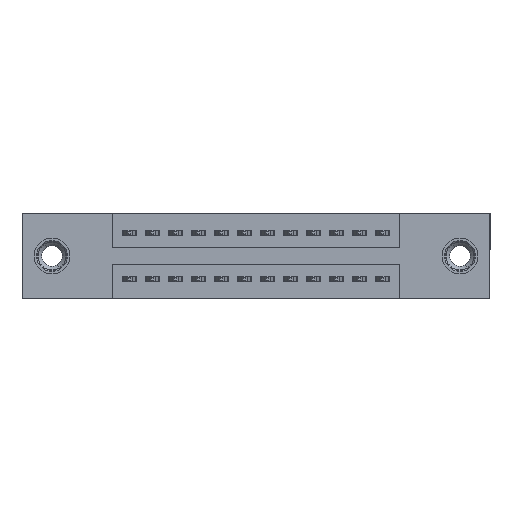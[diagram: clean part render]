
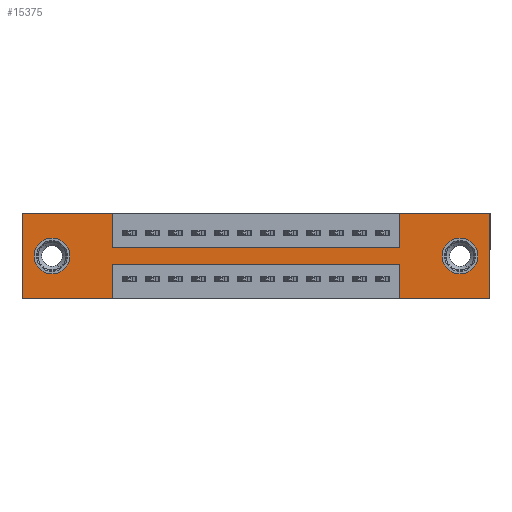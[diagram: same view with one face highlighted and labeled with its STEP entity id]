
A CAD part, front view. The second image highlights one B-rep face of the part: STEP entity #15375.
In plain terms, the highlighted planar face has unit normal (0, -1, 0).
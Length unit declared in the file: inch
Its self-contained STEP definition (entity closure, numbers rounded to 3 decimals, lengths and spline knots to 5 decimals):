
#65 = DIRECTION ( 'NONE',  ( -1., 0., 0. ) ) ;
#118 = ORIENTED_EDGE ( 'NONE', *, *, #15024, .F. ) ;
#172 = AXIS2_PLACEMENT_3D ( 'NONE', #2912, #1698, #9025 ) ;
#315 = VECTOR ( 'NONE', #1634, 39.37008 ) ;
#339 = VERTEX_POINT ( 'NONE', #6235 ) ;
#439 = ORIENTED_EDGE ( 'NONE', *, *, #13453, .T. ) ;
#585 = EDGE_CURVE ( 'NONE', #5337, #15615, #1363, .T. ) ;
#677 = DIRECTION ( 'NONE',  ( 0., 1., 0. ) ) ;
#715 = DIRECTION ( 'NONE',  ( 0., -1., 0. ) ) ;
#903 = VERTEX_POINT ( 'NONE', #2803 ) ;
#1064 = VERTEX_POINT ( 'NONE', #2848 ) ;
#1244 = ORIENTED_EDGE ( 'NONE', *, *, #11249, .F. ) ;
#1256 = LINE ( 'NONE', #8473, #9997 ) ;
#1363 = CIRCLE ( 'NONE', #172, 0.078 ) ;
#1538 = VECTOR ( 'NONE', #12690, 39.37008 ) ;
#1634 = DIRECTION ( 'NONE',  ( -1., 0., 0. ) ) ;
#1678 = CARTESIAN_POINT ( 'NONE',  ( 0.13, 0., -0.185 ) ) ;
#1698 = DIRECTION ( 'NONE',  ( 0., 1., 0. ) ) ;
#1923 = DIRECTION ( 'NONE',  ( 0., 0., -1. ) ) ;
#1973 = EDGE_CURVE ( 'NONE', #9704, #10598, #13847, .T. ) ;
#2004 = VERTEX_POINT ( 'NONE', #6261 ) ;
#2023 = ORIENTED_EDGE ( 'NONE', *, *, #9895, .F. ) ;
#2038 = LINE ( 'NONE', #3874, #14776 ) ;
#2069 = CARTESIAN_POINT ( 'NONE',  ( 0.3925, 0., 0. ) ) ;
#2102 = VECTOR ( 'NONE', #7076, 39.37008 ) ;
#2186 = EDGE_LOOP ( 'NONE', ( #14781, #3223 ) ) ;
#2247 = VECTOR ( 'NONE', #9769, 39.37008 ) ;
#2289 = DIRECTION ( 'NONE',  ( 0., 0., -1. ) ) ;
#2342 = CARTESIAN_POINT ( 'NONE',  ( 0., 0., 0. ) ) ;
#2355 = VERTEX_POINT ( 'NONE', #6116 ) ;
#2509 = VERTEX_POINT ( 'NONE', #3769 ) ;
#2595 = DIRECTION ( 'NONE',  ( 0., 0., 1. ) ) ;
#2657 = FACE_BOUND ( 'NONE', #2186, .T. ) ;
#2741 = CARTESIAN_POINT ( 'NONE',  ( 0.3925, 0., -0.22 ) ) ;
#2803 = CARTESIAN_POINT ( 'NONE',  ( 2.035, 0., 0. ) ) ;
#2838 = ORIENTED_EDGE ( 'NONE', *, *, #7203, .F. ) ;
#2848 = CARTESIAN_POINT ( 'NONE',  ( 1.6425, 0., -0.37 ) ) ;
#2882 = DIRECTION ( 'NONE',  ( 0., 0., 1. ) ) ;
#2912 = CARTESIAN_POINT ( 'NONE',  ( 1.905, 0., -0.185 ) ) ;
#3102 = DIRECTION ( 'NONE',  ( 0., 0., -1. ) ) ;
#3210 = CARTESIAN_POINT ( 'NONE',  ( 1.905, 0., -0.107 ) ) ;
#3223 = ORIENTED_EDGE ( 'NONE', *, *, #9840, .T. ) ;
#3570 = CARTESIAN_POINT ( 'NONE',  ( 0.3925, 0., -0.15 ) ) ;
#3715 = VERTEX_POINT ( 'NONE', #8625 ) ;
#3760 = LINE ( 'NONE', #9554, #12488 ) ;
#3769 = CARTESIAN_POINT ( 'NONE',  ( 0., 0., -0.37 ) ) ;
#3874 = CARTESIAN_POINT ( 'NONE',  ( 0.3925, 0., 0. ) ) ;
#4836 = CARTESIAN_POINT ( 'NONE',  ( 0.13, 0., -0.185 ) ) ;
#4933 = ORIENTED_EDGE ( 'NONE', *, *, #10602, .F. ) ;
#5054 = LINE ( 'NONE', #15081, #10585 ) ;
#5174 = CARTESIAN_POINT ( 'NONE',  ( 1.6425, 0., 0. ) ) ;
#5337 = VERTEX_POINT ( 'NONE', #3210 ) ;
#5484 = VECTOR ( 'NONE', #6401, 39.37008 ) ;
#5520 = VERTEX_POINT ( 'NONE', #2069 ) ;
#5568 = EDGE_LOOP ( 'NONE', ( #14565, #2838, #118, #6949, #2023, #13502, #9833, #5619, #14985, #7080, #4933, #1244 ) ) ;
#5619 = ORIENTED_EDGE ( 'NONE', *, *, #14293, .F. ) ;
#5626 = VECTOR ( 'NONE', #65, 39.37008 ) ;
#6069 = AXIS2_PLACEMENT_3D ( 'NONE', #4836, #14409, #7340 ) ;
#6116 = CARTESIAN_POINT ( 'NONE',  ( 1.6425, 0., -0.22 ) ) ;
#6183 = DIRECTION ( 'NONE',  ( 0., 0., 1. ) ) ;
#6235 = CARTESIAN_POINT ( 'NONE',  ( 0., 0., 0. ) ) ;
#6252 = LINE ( 'NONE', #12428, #5484 ) ;
#6261 = CARTESIAN_POINT ( 'NONE',  ( 0.3925, 0., -0.37 ) ) ;
#6304 = CARTESIAN_POINT ( 'NONE',  ( 0., 0., -0.37 ) ) ;
#6401 = DIRECTION ( 'NONE',  ( 1., 0., 0. ) ) ;
#6461 = CARTESIAN_POINT ( 'NONE',  ( 1.6425, 0., -0.15 ) ) ;
#6746 = CARTESIAN_POINT ( 'NONE',  ( 2.035, 0., -0.37 ) ) ;
#6843 = FACE_BOUND ( 'NONE', #10424, .T. ) ;
#6949 = ORIENTED_EDGE ( 'NONE', *, *, #10129, .F. ) ;
#7076 = DIRECTION ( 'NONE',  ( 0., 0., 1. ) ) ;
#7080 = ORIENTED_EDGE ( 'NONE', *, *, #14632, .F. ) ;
#7122 = CARTESIAN_POINT ( 'NONE',  ( 0.13, 0., -0.263 ) ) ;
#7203 = EDGE_CURVE ( 'NONE', #2355, #14666, #13108, .T. ) ;
#7340 = DIRECTION ( 'NONE',  ( 0., 0., 1. ) ) ;
#7537 = CARTESIAN_POINT ( 'NONE',  ( 0., 0., -0.37 ) ) ;
#7743 = CIRCLE ( 'NONE', #13433, 0.078 ) ;
#7795 = CARTESIAN_POINT ( 'NONE',  ( 1.905, 0., -0.185 ) ) ;
#7968 = CARTESIAN_POINT ( 'NONE',  ( 0., 0., -0.37 ) ) ;
#8262 = AXIS2_PLACEMENT_3D ( 'NONE', #7968, #715, #1923 ) ;
#8446 = VERTEX_POINT ( 'NONE', #6746 ) ;
#8473 = CARTESIAN_POINT ( 'NONE',  ( 0., 0., 0. ) ) ;
#8625 = CARTESIAN_POINT ( 'NONE',  ( 0.3925, 0., -0.15 ) ) ;
#8659 = EDGE_CURVE ( 'NONE', #5520, #3715, #2038, .T. ) ;
#8688 = EDGE_CURVE ( 'NONE', #14666, #2004, #3760, .T. ) ;
#8820 = VERTEX_POINT ( 'NONE', #12036 ) ;
#8821 = EDGE_CURVE ( 'NONE', #10598, #903, #14568, .T. ) ;
#9025 = DIRECTION ( 'NONE',  ( 0., 0., -1. ) ) ;
#9554 = CARTESIAN_POINT ( 'NONE',  ( 0.3925, 0., -0.37 ) ) ;
#9704 = VERTEX_POINT ( 'NONE', #6461 ) ;
#9769 = DIRECTION ( 'NONE',  ( 1., 0., 0. ) ) ;
#9833 = ORIENTED_EDGE ( 'NONE', *, *, #1973, .F. ) ;
#9840 = EDGE_CURVE ( 'NONE', #15615, #5337, #7743, .T. ) ;
#9895 = EDGE_CURVE ( 'NONE', #903, #8446, #5054, .T. ) ;
#9997 = VECTOR ( 'NONE', #6183, 39.37008 ) ;
#10129 = EDGE_CURVE ( 'NONE', #8446, #1064, #14146, .T. ) ;
#10424 = EDGE_LOOP ( 'NONE', ( #439, #11477 ) ) ;
#10585 = VECTOR ( 'NONE', #11647, 39.37008 ) ;
#10598 = VERTEX_POINT ( 'NONE', #14524 ) ;
#10602 = EDGE_CURVE ( 'NONE', #2509, #339, #1256, .T. ) ;
#11003 = DIRECTION ( 'NONE',  ( 0., 0., -1. ) ) ;
#11249 = EDGE_CURVE ( 'NONE', #2004, #2509, #12061, .T. ) ;
#11477 = ORIENTED_EDGE ( 'NONE', *, *, #14800, .T. ) ;
#11647 = DIRECTION ( 'NONE',  ( 0., 0., -1. ) ) ;
#11784 = LINE ( 'NONE', #15614, #2102 ) ;
#12036 = CARTESIAN_POINT ( 'NONE',  ( 0.13, 0., -0.107 ) ) ;
#12061 = LINE ( 'NONE', #6304, #315 ) ;
#12258 = CARTESIAN_POINT ( 'NONE',  ( 0.3925, 0., -0.22 ) ) ;
#12348 = VECTOR ( 'NONE', #2595, 39.37008 ) ;
#12428 = CARTESIAN_POINT ( 'NONE',  ( 0., 0., 0. ) ) ;
#12488 = VECTOR ( 'NONE', #2289, 39.37008 ) ;
#12690 = DIRECTION ( 'NONE',  ( 1., 0., 0. ) ) ;
#12798 = VERTEX_POINT ( 'NONE', #7122 ) ;
#13108 = LINE ( 'NONE', #12258, #15554 ) ;
#13433 = AXIS2_PLACEMENT_3D ( 'NONE', #7795, #677, #3102 ) ;
#13453 = EDGE_CURVE ( 'NONE', #8820, #12798, #13839, .T. ) ;
#13502 = ORIENTED_EDGE ( 'NONE', *, *, #8821, .F. ) ;
#13633 = FACE_OUTER_BOUND ( 'NONE', #5568, .T. ) ;
#13833 = DIRECTION ( 'NONE',  ( 0., 1., 0. ) ) ;
#13839 = CIRCLE ( 'NONE', #6069, 0.078 ) ;
#13847 = LINE ( 'NONE', #5174, #12348 ) ;
#14146 = LINE ( 'NONE', #7537, #5626 ) ;
#14186 = CARTESIAN_POINT ( 'NONE',  ( 1.905, 0., -0.263 ) ) ;
#14293 = EDGE_CURVE ( 'NONE', #3715, #9704, #14389, .T. ) ;
#14389 = LINE ( 'NONE', #3570, #1538 ) ;
#14409 = DIRECTION ( 'NONE',  ( 0., 1., 0. ) ) ;
#14524 = CARTESIAN_POINT ( 'NONE',  ( 1.6425, 0., 0. ) ) ;
#14565 = ORIENTED_EDGE ( 'NONE', *, *, #8688, .F. ) ;
#14568 = LINE ( 'NONE', #2342, #2247 ) ;
#14632 = EDGE_CURVE ( 'NONE', #339, #5520, #6252, .T. ) ;
#14666 = VERTEX_POINT ( 'NONE', #2741 ) ;
#14776 = VECTOR ( 'NONE', #11003, 39.37008 ) ;
#14781 = ORIENTED_EDGE ( 'NONE', *, *, #585, .T. ) ;
#14800 = EDGE_CURVE ( 'NONE', #12798, #8820, #15151, .T. ) ;
#14849 = DIRECTION ( 'NONE',  ( -1., 0., 0. ) ) ;
#14907 = AXIS2_PLACEMENT_3D ( 'NONE', #1678, #13833, #2882 ) ;
#14985 = ORIENTED_EDGE ( 'NONE', *, *, #8659, .F. ) ;
#15024 = EDGE_CURVE ( 'NONE', #1064, #2355, #11784, .T. ) ;
#15081 = CARTESIAN_POINT ( 'NONE',  ( 2.035, 0., 0. ) ) ;
#15151 = CIRCLE ( 'NONE', #14907, 0.078 ) ;
#15221 = PLANE ( 'NONE',  #8262 ) ;
#15375 = ADVANCED_FACE ( 'NONE', ( #2657, #6843, #13633 ), #15221, .T. ) ;
#15554 = VECTOR ( 'NONE', #14849, 39.37008 ) ;
#15614 = CARTESIAN_POINT ( 'NONE',  ( 1.6425, 0., -0.37 ) ) ;
#15615 = VERTEX_POINT ( 'NONE', #14186 ) ;
